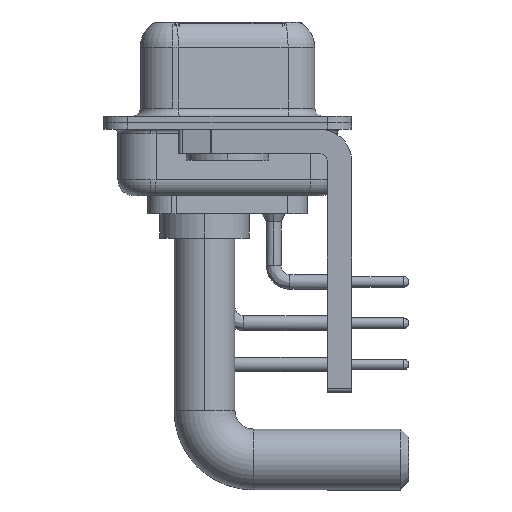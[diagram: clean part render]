
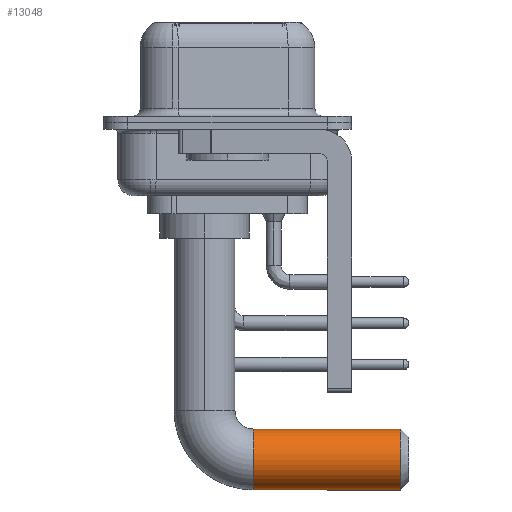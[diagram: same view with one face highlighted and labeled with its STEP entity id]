
A CAD part, left-side view. The second image highlights one B-rep face of the part: STEP entity #13048.
In plain terms, the highlighted cylindrical face has radius 1.875 mm (diameter 3.75 mm), a partial arc.
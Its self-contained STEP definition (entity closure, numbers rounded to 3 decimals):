
#999 = ORIENTED_EDGE ( 'NONE', *, *, #23421, .T. ) ;
#1890 = ORIENTED_EDGE ( 'NONE', *, *, #26696, .T. ) ;
#2374 = ORIENTED_EDGE ( 'NONE', *, *, #11237, .F. ) ;
#3195 = CARTESIAN_POINT ( 'NONE',  ( 0., -12.07, -13.63 ) ) ;
#5763 = CARTESIAN_POINT ( 'NONE',  ( 0., -3., -15.505 ) ) ;
#5881 = LINE ( 'NONE', #21499, #18327 ) ;
#6056 = DIRECTION ( 'NONE',  ( 0., -1., 0. ) ) ;
#7832 = AXIS2_PLACEMENT_3D ( 'NONE', #3195, #13896, #30229 ) ;
#7900 = DIRECTION ( 'NONE',  ( -1., 0., 0. ) ) ;
#7984 = VERTEX_POINT ( 'NONE', #30132 ) ;
#8647 = ORIENTED_EDGE ( 'NONE', *, *, #21995, .T. ) ;
#11191 = LINE ( 'NONE', #5763, #23752 ) ;
#11237 = EDGE_CURVE ( 'NONE', #29474, #7984, #5881, .T. ) ;
#13048 = ADVANCED_FACE ( 'NONE', ( #17111 ), #14476, .T. ) ;
#13744 = CARTESIAN_POINT ( 'NONE',  ( 0., -3., -15.505 ) ) ;
#13896 = DIRECTION ( 'NONE',  ( 0., 1., 0. ) ) ;
#14476 = CYLINDRICAL_SURFACE ( 'NONE', #31926, 1.875 ) ;
#15647 = CIRCLE ( 'NONE', #30830, 1.875 ) ;
#15957 = DIRECTION ( 'NONE',  ( 0., -1., 0. ) ) ;
#16619 = CARTESIAN_POINT ( 'NONE',  ( 0., -12.07, -15.505 ) ) ;
#17111 = FACE_OUTER_BOUND ( 'NONE', #29766, .T. ) ;
#18327 = VECTOR ( 'NONE', #6056, 1000. ) ;
#21499 = CARTESIAN_POINT ( 'NONE',  ( 0., -3., -11.755 ) ) ;
#21995 = EDGE_CURVE ( 'NONE', #29474, #26158, #15647, .T. ) ;
#22268 = DIRECTION ( 'NONE',  ( 0., -1., 0. ) ) ;
#23421 = EDGE_CURVE ( 'NONE', #32394, #7984, #30827, .T. ) ;
#23752 = VECTOR ( 'NONE', #22268, 1000. ) ;
#23884 = CARTESIAN_POINT ( 'NONE',  ( 0., -3., -13.63 ) ) ;
#25228 = DIRECTION ( 'NONE',  ( 0., 0., -1. ) ) ;
#26158 = VERTEX_POINT ( 'NONE', #13744 ) ;
#26696 = EDGE_CURVE ( 'NONE', #26158, #32394, #11191, .T. ) ;
#27813 = CARTESIAN_POINT ( 'NONE',  ( 0., -3., -11.755 ) ) ;
#27857 = DIRECTION ( 'NONE',  ( 0., -1., 0. ) ) ;
#29474 = VERTEX_POINT ( 'NONE', #27813 ) ;
#29766 = EDGE_LOOP ( 'NONE', ( #2374, #8647, #1890, #999 ) ) ;
#30132 = CARTESIAN_POINT ( 'NONE',  ( 0., -12.07, -11.755 ) ) ;
#30229 = DIRECTION ( 'NONE',  ( 0., 0., -1. ) ) ;
#30827 = CIRCLE ( 'NONE', #7832, 1.875 ) ;
#30830 = AXIS2_PLACEMENT_3D ( 'NONE', #23884, #15957, #7900 ) ;
#31926 = AXIS2_PLACEMENT_3D ( 'NONE', #32583, #27857, #25228 ) ;
#32394 = VERTEX_POINT ( 'NONE', #16619 ) ;
#32583 = CARTESIAN_POINT ( 'NONE',  ( 0., -3., -13.63 ) ) ;
